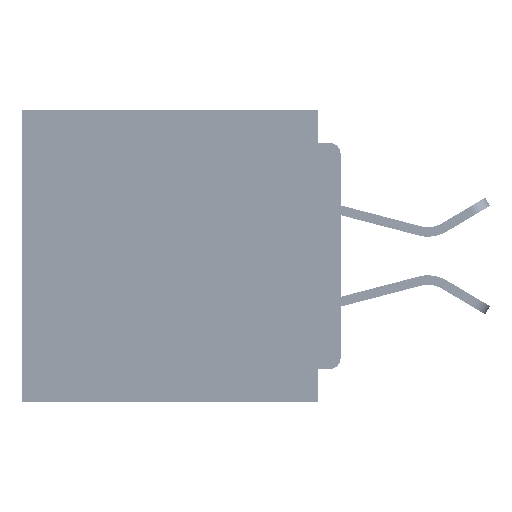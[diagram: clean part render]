
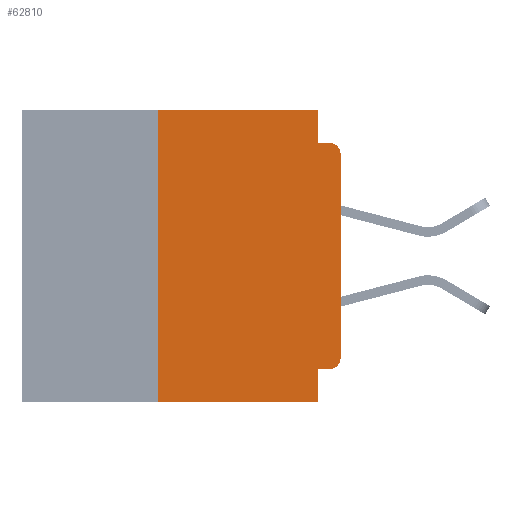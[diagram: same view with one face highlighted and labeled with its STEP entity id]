
A CAD part, left-side view. The second image highlights one B-rep face of the part: STEP entity #62810.
In plain terms, the highlighted planar face has unit normal (-1, 0, 0).
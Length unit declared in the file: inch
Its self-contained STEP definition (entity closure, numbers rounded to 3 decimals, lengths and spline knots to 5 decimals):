
#1294 = VERTEX_POINT ( 'NONE', #38178 ) ;
#1866 = ORIENTED_EDGE ( 'NONE', *, *, #42277, .T. ) ;
#2404 = CARTESIAN_POINT ( 'NONE',  ( 0., 0.015, -0.355 ) ) ;
#2728 = EDGE_CURVE ( 'NONE', #1294, #17852, #38336, .T. ) ;
#2878 = DIRECTION ( 'NONE',  ( 0., 1., 0. ) ) ;
#4201 = VERTEX_POINT ( 'NONE', #61276 ) ;
#4446 = EDGE_LOOP ( 'NONE', ( #1866, #47105, #10388, #25128, #9462, #28078, #63664, #54563, #59897, #9065 ) ) ;
#5071 = VERTEX_POINT ( 'NONE', #8105 ) ;
#5316 = EDGE_CURVE ( 'NONE', #11651, #34231, #29269, .T. ) ;
#5472 = CARTESIAN_POINT ( 'NONE',  ( 0., 0.25, -0.4 ) ) ;
#8105 = CARTESIAN_POINT ( 'NONE',  ( 0., 0.031, -0.355 ) ) ;
#9065 = ORIENTED_EDGE ( 'NONE', *, *, #11142, .T. ) ;
#9462 = ORIENTED_EDGE ( 'NONE', *, *, #5316, .F. ) ;
#10388 = ORIENTED_EDGE ( 'NONE', *, *, #41395, .F. ) ;
#11142 = EDGE_CURVE ( 'NONE', #14892, #34314, #52956, .T. ) ;
#11196 = CARTESIAN_POINT ( 'NONE',  ( 0., 0.031, -0.4 ) ) ;
#11651 = VERTEX_POINT ( 'NONE', #55496 ) ;
#11776 = CARTESIAN_POINT ( 'NONE',  ( 0., 0.437, 0. ) ) ;
#12625 = CARTESIAN_POINT ( 'NONE',  ( 0., 0., -0.045 ) ) ;
#14315 = CARTESIAN_POINT ( 'NONE',  ( 0., 0., 0. ) ) ;
#14714 = VECTOR ( 'NONE', #38659, 39.37008 ) ;
#14892 = VERTEX_POINT ( 'NONE', #2404 ) ;
#16274 = CARTESIAN_POINT ( 'NONE',  ( 0., 0.015, -0.34 ) ) ;
#17852 = VERTEX_POINT ( 'NONE', #45620 ) ;
#21350 = DIRECTION ( 'NONE',  ( 0., 0., -1. ) ) ;
#21437 = VERTEX_POINT ( 'NONE', #61902 ) ;
#25116 = LINE ( 'NONE', #11196, #65404 ) ;
#25128 = ORIENTED_EDGE ( 'NONE', *, *, #26804, .F. ) ;
#26804 = EDGE_CURVE ( 'NONE', #34231, #21437, #33000, .T. ) ;
#26827 = PLANE ( 'NONE',  #62029 ) ;
#27035 = DIRECTION ( 'NONE',  ( 1., 0., 0. ) ) ;
#27171 = CARTESIAN_POINT ( 'NONE',  ( 0., 0.25, -0.4 ) ) ;
#27672 = VECTOR ( 'NONE', #45505, 39.37008 ) ;
#28078 = ORIENTED_EDGE ( 'NONE', *, *, #61590, .F. ) ;
#28132 = LINE ( 'NONE', #58532, #53399 ) ;
#28246 = VECTOR ( 'NONE', #65220, 39.37008 ) ;
#29269 = LINE ( 'NONE', #50552, #27672 ) ;
#29731 = LINE ( 'NONE', #33540, #14714 ) ;
#32583 = EDGE_CURVE ( 'NONE', #34760, #4201, #29731, .T. ) ;
#32639 = FACE_OUTER_BOUND ( 'NONE', #4446, .T. ) ;
#33000 = LINE ( 'NONE', #45121, #28246 ) ;
#33540 = CARTESIAN_POINT ( 'NONE',  ( 0., 0.437, -0.4 ) ) ;
#34231 = VERTEX_POINT ( 'NONE', #62032 ) ;
#34314 = VERTEX_POINT ( 'NONE', #57380 ) ;
#34563 = VECTOR ( 'NONE', #58121, 39.37008 ) ;
#34642 = DIRECTION ( 'NONE',  ( 0., 0., 1. ) ) ;
#34760 = VERTEX_POINT ( 'NONE', #5472 ) ;
#36399 = AXIS2_PLACEMENT_3D ( 'NONE', #48160, #48006, #47934 ) ;
#38178 = CARTESIAN_POINT ( 'NONE',  ( 0., 0., -0.06 ) ) ;
#38336 = CIRCLE ( 'NONE', #36399, 0.015 ) ;
#38659 = DIRECTION ( 'NONE',  ( 0., -1., 0. ) ) ;
#40608 = VECTOR ( 'NONE', #57402, 39.37008 ) ;
#41100 = VECTOR ( 'NONE', #34642, 39.37008 ) ;
#41395 = EDGE_CURVE ( 'NONE', #21437, #17852, #48024, .T. ) ;
#42277 = EDGE_CURVE ( 'NONE', #34314, #1294, #42725, .T. ) ;
#42725 = LINE ( 'NONE', #14315, #41100 ) ;
#45121 = CARTESIAN_POINT ( 'NONE',  ( 0., 0.031, 0. ) ) ;
#45339 = EDGE_CURVE ( 'NONE', #14892, #5071, #28132, .T. ) ;
#45505 = DIRECTION ( 'NONE',  ( 0., -1., 0. ) ) ;
#45620 = CARTESIAN_POINT ( 'NONE',  ( 0., 0.015, -0.045 ) ) ;
#46602 = DIRECTION ( 'NONE',  ( 0., 0., -1. ) ) ;
#47105 = ORIENTED_EDGE ( 'NONE', *, *, #2728, .T. ) ;
#47934 = DIRECTION ( 'NONE',  ( 0., 0., -1. ) ) ;
#48006 = DIRECTION ( 'NONE',  ( -1., 0., 0. ) ) ;
#48024 = LINE ( 'NONE', #12625, #34563 ) ;
#48160 = CARTESIAN_POINT ( 'NONE',  ( 0., 0.015, -0.06 ) ) ;
#50552 = CARTESIAN_POINT ( 'NONE',  ( 0., 0.437, 0. ) ) ;
#51575 = DIRECTION ( 'NONE',  ( -1., 0., 0. ) ) ;
#52429 = LINE ( 'NONE', #27171, #40608 ) ;
#52956 = CIRCLE ( 'NONE', #62514, 0.015 ) ;
#53399 = VECTOR ( 'NONE', #2878, 39.37008 ) ;
#54563 = ORIENTED_EDGE ( 'NONE', *, *, #60262, .F. ) ;
#55496 = CARTESIAN_POINT ( 'NONE',  ( 0., 0.25, 0. ) ) ;
#57380 = CARTESIAN_POINT ( 'NONE',  ( 0., 0., -0.34 ) ) ;
#57402 = DIRECTION ( 'NONE',  ( 0., 0., 1. ) ) ;
#58121 = DIRECTION ( 'NONE',  ( 0., -1., 0. ) ) ;
#58532 = CARTESIAN_POINT ( 'NONE',  ( 0., 0., -0.355 ) ) ;
#59897 = ORIENTED_EDGE ( 'NONE', *, *, #45339, .F. ) ;
#60262 = EDGE_CURVE ( 'NONE', #5071, #4201, #25116, .T. ) ;
#61276 = CARTESIAN_POINT ( 'NONE',  ( 0., 0.031, -0.4 ) ) ;
#61590 = EDGE_CURVE ( 'NONE', #34760, #11651, #52429, .T. ) ;
#61902 = CARTESIAN_POINT ( 'NONE',  ( 0., 0.031, -0.045 ) ) ;
#62029 = AXIS2_PLACEMENT_3D ( 'NONE', #11776, #27035, #62366 ) ;
#62032 = CARTESIAN_POINT ( 'NONE',  ( 0., 0.031, 0. ) ) ;
#62366 = DIRECTION ( 'NONE',  ( 0., 0., -1. ) ) ;
#62514 = AXIS2_PLACEMENT_3D ( 'NONE', #16274, #51575, #21350 ) ;
#62810 = ADVANCED_FACE ( 'NONE', ( #32639 ), #26827, .F. ) ;
#63664 = ORIENTED_EDGE ( 'NONE', *, *, #32583, .T. ) ;
#65220 = DIRECTION ( 'NONE',  ( 0., 0., -1. ) ) ;
#65404 = VECTOR ( 'NONE', #46602, 39.37008 ) ;
